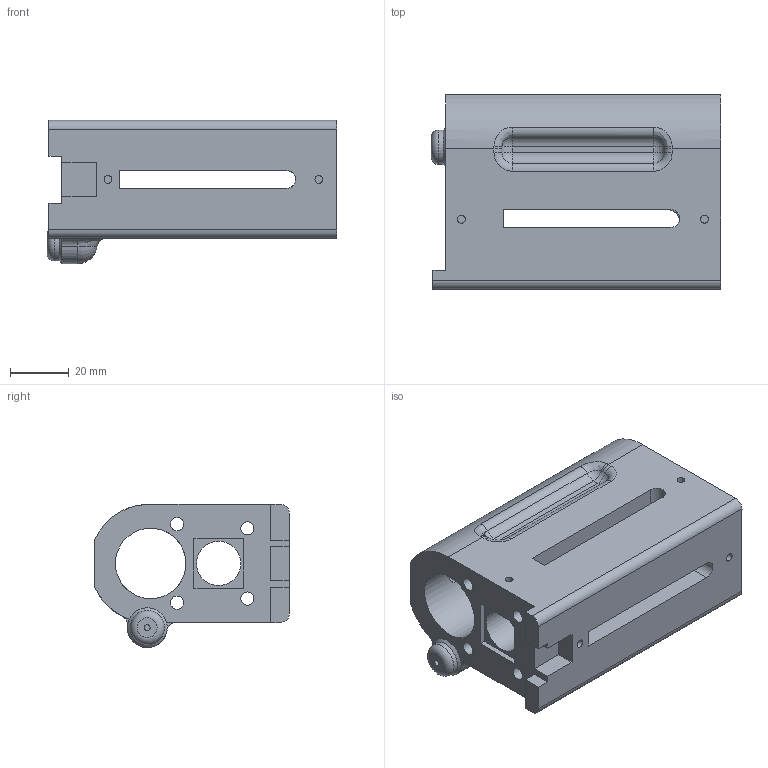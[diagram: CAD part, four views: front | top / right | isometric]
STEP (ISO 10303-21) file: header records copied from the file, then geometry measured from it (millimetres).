
FILE_DESCRIPTION (( 'STEP AP203' ), '1' );
FILE_NAME ('handguard.STEP', '2020-05-10T06:14:24', ( '' ), ( '' ), 'SwSTEP 2.0', 'SolidWorks 2016', '' );
FILE_SCHEMA (( 'CONFIG_CONTROL_DESIGN' ));
Length unit declared in the file: millimetre
Products named in the file (1): handguard
Bounding box: 98.62 x 66.17 x 48.74 mm (x, y, z)
Volume: 131206.4 mm3; surface area: 42993.3 mm2
Topology: 1 solids, 2 shells, 179 faces, 442 edges, 273 vertices
Faces by surface type: cylinder 66, plane 59, bspline 22, torus 19, sphere 12, cone 1
Full cylindrical faces by diameter (mm): 2 x1, 2.7 x6, 4.5 x4, 11.7 x1, 15.1 x1, 20.5 x1, 24 x1
Entity records: 6463 total; most frequent: CARTESIAN_POINT 2343, ORIENTED_EDGE 844, DIRECTION 793, EDGE_CURVE 422, AXIS2_PLACEMENT_3D 305, VERTEX_POINT 270, EDGE_LOOP 224, FACE_OUTER_BOUND 195
